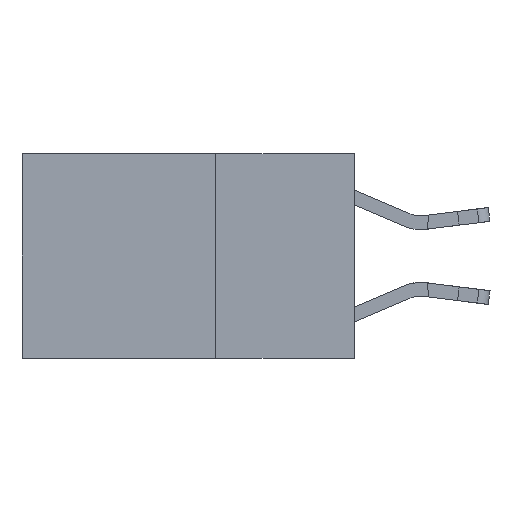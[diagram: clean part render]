
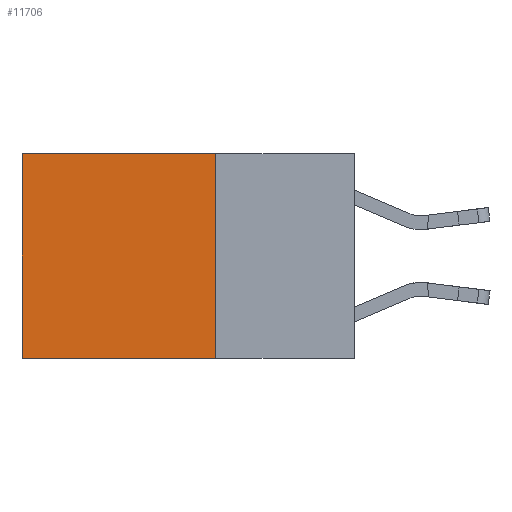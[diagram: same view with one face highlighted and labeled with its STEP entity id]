
A CAD part, left-side view. The second image highlights one B-rep face of the part: STEP entity #11706.
In plain terms, the highlighted planar face has unit normal (-1, 0, 0).
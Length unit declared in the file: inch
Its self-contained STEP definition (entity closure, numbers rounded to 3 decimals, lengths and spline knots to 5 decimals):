
#642 = VECTOR ( 'NONE', #12732, 39.37008 ) ;
#2335 = CARTESIAN_POINT ( 'NONE',  ( 0.2625, 0.6, 0. ) ) ;
#3208 = ORIENTED_EDGE ( 'NONE', *, *, #6067, .F. ) ;
#3275 = ORIENTED_EDGE ( 'NONE', *, *, #16940, .T. ) ;
#3473 = CARTESIAN_POINT ( 'NONE',  ( 0.2625, 0.6, -0.37 ) ) ;
#4426 = CARTESIAN_POINT ( 'NONE',  ( 0.2625, 0.25, -0.37 ) ) ;
#4563 = LINE ( 'NONE', #10382, #9444 ) ;
#5849 = ORIENTED_EDGE ( 'NONE', *, *, #19453, .F. ) ;
#5864 = PLANE ( 'NONE',  #13140 ) ;
#6067 = EDGE_CURVE ( 'NONE', #15789, #13003, #17275, .T. ) ;
#6315 = VECTOR ( 'NONE', #11870, 39.37008 ) ;
#6576 = FACE_OUTER_BOUND ( 'NONE', #9839, .T. ) ;
#6745 = VERTEX_POINT ( 'NONE', #7827 ) ;
#6996 = EDGE_CURVE ( 'NONE', #26316, #13003, #22754, .T. ) ;
#7827 = CARTESIAN_POINT ( 'NONE',  ( 0.2625, 0.25, 0. ) ) ;
#7941 = CARTESIAN_POINT ( 'NONE',  ( 0.2625, 0.25, 0. ) ) ;
#9273 = ORIENTED_EDGE ( 'NONE', *, *, #6996, .T. ) ;
#9444 = VECTOR ( 'NONE', #20657, 39.37008 ) ;
#9629 = VECTOR ( 'NONE', #15925, 39.37008 ) ;
#9839 = EDGE_LOOP ( 'NONE', ( #9273, #3208, #5849, #3275 ) ) ;
#10039 = DIRECTION ( 'NONE',  ( 1., 0., 0. ) ) ;
#10382 = CARTESIAN_POINT ( 'NONE',  ( 0.2625, 0.25, 0. ) ) ;
#11706 = ADVANCED_FACE ( 'NONE', ( #6576 ), #5864, .F. ) ;
#11870 = DIRECTION ( 'NONE',  ( 0., 1., 0. ) ) ;
#12732 = DIRECTION ( 'NONE',  ( 0., 0., -1. ) ) ;
#13003 = VERTEX_POINT ( 'NONE', #3473 ) ;
#13140 = AXIS2_PLACEMENT_3D ( 'NONE', #7941, #10039, #24475 ) ;
#13950 = CARTESIAN_POINT ( 'NONE',  ( 0.2625, 0.25, -0.37 ) ) ;
#15789 = VERTEX_POINT ( 'NONE', #4426 ) ;
#15925 = DIRECTION ( 'NONE',  ( 0., 0., -1. ) ) ;
#16940 = EDGE_CURVE ( 'NONE', #6745, #26316, #4563, .T. ) ;
#17275 = LINE ( 'NONE', #13950, #6315 ) ;
#19453 = EDGE_CURVE ( 'NONE', #6745, #15789, #26083, .T. ) ;
#20657 = DIRECTION ( 'NONE',  ( 0., 1., 0. ) ) ;
#22754 = LINE ( 'NONE', #2335, #642 ) ;
#24146 = CARTESIAN_POINT ( 'NONE',  ( 0.2625, 0.25, 0. ) ) ;
#24475 = DIRECTION ( 'NONE',  ( 0., 0., -1. ) ) ;
#25082 = CARTESIAN_POINT ( 'NONE',  ( 0.2625, 0.6, 0. ) ) ;
#26083 = LINE ( 'NONE', #24146, #9629 ) ;
#26316 = VERTEX_POINT ( 'NONE', #25082 ) ;
